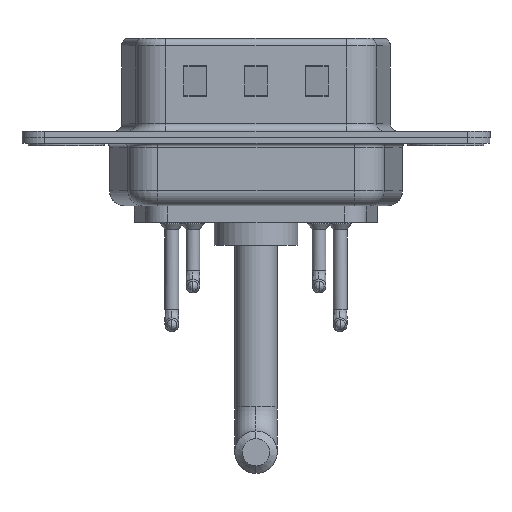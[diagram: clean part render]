
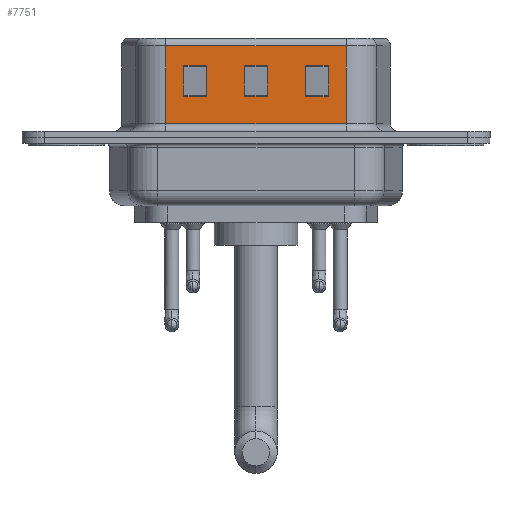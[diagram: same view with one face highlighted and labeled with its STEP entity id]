
A CAD part, front view. The second image highlights one B-rep face of the part: STEP entity #7751.
In plain terms, the highlighted planar face has unit normal (0, -1, 0).
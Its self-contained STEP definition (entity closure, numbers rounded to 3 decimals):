
#421 = FACE_OUTER_BOUND ( 'NONE', #4052, .T. ) ;
#443 = LINE ( 'NONE', #3207, #544 ) ;
#544 = VECTOR ( 'NONE', #8611, 1000. ) ;
#667 = CARTESIAN_POINT ( 'NONE',  ( 7.75, -4.55, 2.705 ) ) ;
#671 = EDGE_CURVE ( 'NONE', #2100, #13648, #8820, .T. ) ;
#687 = DIRECTION ( 'NONE',  ( -1., 0., 0. ) ) ;
#798 = CARTESIAN_POINT ( 'NONE',  ( 11.75, -4.55, 2.705 ) ) ;
#935 = VERTEX_POINT ( 'NONE', #10916 ) ;
#1129 = EDGE_CURVE ( 'NONE', #3249, #13565, #11457, .T. ) ;
#1259 = VECTOR ( 'NONE', #13180, 1000. ) ;
#1276 = CARTESIAN_POINT ( 'NONE',  ( 18.451, -4.55, 6.02 ) ) ;
#1344 = VECTOR ( 'NONE', #3215, 1000. ) ;
#1356 = DIRECTION ( 'NONE',  ( 1., 0., 0. ) ) ;
#1437 = VERTEX_POINT ( 'NONE', #798 ) ;
#1590 = VERTEX_POINT ( 'NONE', #16400 ) ;
#1668 = FACE_BOUND ( 'NONE', #7060, .T. ) ;
#1774 = VERTEX_POINT ( 'NONE', #2992 ) ;
#1890 = EDGE_CURVE ( 'NONE', #15022, #1437, #7708, .T. ) ;
#1891 = EDGE_CURVE ( 'NONE', #13648, #3902, #11852, .T. ) ;
#2100 = VERTEX_POINT ( 'NONE', #8487 ) ;
#2516 = CARTESIAN_POINT ( 'NONE',  ( 14.451, -4.55, 4.705 ) ) ;
#2557 = EDGE_CURVE ( 'NONE', #2567, #9146, #14046, .T. ) ;
#2567 = VERTEX_POINT ( 'NONE', #9972 ) ;
#2642 = ORIENTED_EDGE ( 'NONE', *, *, #10683, .T. ) ;
#2862 = ORIENTED_EDGE ( 'NONE', *, *, #17486, .T. ) ;
#2992 = CARTESIAN_POINT ( 'NONE',  ( 15.75, -4.55, 2.705 ) ) ;
#3095 = CARTESIAN_POINT ( 'NONE',  ( 18.451, -4.55, 6.52 ) ) ;
#3207 = CARTESIAN_POINT ( 'NONE',  ( 18.451, -4.55, 0.9 ) ) ;
#3215 = DIRECTION ( 'NONE',  ( 0., 0., 1. ) ) ;
#3233 = DIRECTION ( 'NONE',  ( 1., 0., 0. ) ) ;
#3249 = VERTEX_POINT ( 'NONE', #9520 ) ;
#3403 = DIRECTION ( 'NONE',  ( 1., 0., 0. ) ) ;
#3591 = VECTOR ( 'NONE', #12811, 1000. ) ;
#3627 = CARTESIAN_POINT ( 'NONE',  ( 18.451, -4.55, 0.9 ) ) ;
#3777 = CARTESIAN_POINT ( 'NONE',  ( 22.451, -4.55, 2.705 ) ) ;
#3902 = VERTEX_POINT ( 'NONE', #11196 ) ;
#4052 = EDGE_LOOP ( 'NONE', ( #14778, #10621, #5900, #13824 ) ) ;
#4196 = VERTEX_POINT ( 'NONE', #8003 ) ;
#4201 = DIRECTION ( 'NONE',  ( 0., 0., -1. ) ) ;
#4216 = ORIENTED_EDGE ( 'NONE', *, *, #14753, .T. ) ;
#4244 = VECTOR ( 'NONE', #3233, 1000. ) ;
#4467 = VECTOR ( 'NONE', #11379, 1000. ) ;
#5243 = DIRECTION ( 'NONE',  ( 0., 0., -1. ) ) ;
#5418 = CARTESIAN_POINT ( 'NONE',  ( 6.549, -4.55, 6.02 ) ) ;
#5514 = LINE ( 'NONE', #2516, #11904 ) ;
#5900 = ORIENTED_EDGE ( 'NONE', *, *, #15663, .T. ) ;
#6039 = ORIENTED_EDGE ( 'NONE', *, *, #11888, .T. ) ;
#6347 = CARTESIAN_POINT ( 'NONE',  ( 11.75, -4.55, 6.52 ) ) ;
#6568 = CARTESIAN_POINT ( 'NONE',  ( 9.25, -4.55, 4.705 ) ) ;
#6750 = CARTESIAN_POINT ( 'NONE',  ( 6.549, -4.55, 6.52 ) ) ;
#6927 = VECTOR ( 'NONE', #687, 1000. ) ;
#7060 = EDGE_LOOP ( 'NONE', ( #4216, #15397, #7158, #9634 ) ) ;
#7158 = ORIENTED_EDGE ( 'NONE', *, *, #12634, .T. ) ;
#7344 = VECTOR ( 'NONE', #10807, 1000. ) ;
#7421 = CARTESIAN_POINT ( 'NONE',  ( 17.25, -4.55, 4.705 ) ) ;
#7506 = ORIENTED_EDGE ( 'NONE', *, *, #9407, .T. ) ;
#7522 = CARTESIAN_POINT ( 'NONE',  ( 13.25, -4.55, 2.705 ) ) ;
#7557 = LINE ( 'NONE', #8884, #10496 ) ;
#7708 = LINE ( 'NONE', #9021, #6927 ) ;
#7721 = EDGE_LOOP ( 'NONE', ( #12800, #2642, #14802, #7990 ) ) ;
#7751 = ADVANCED_FACE ( 'NONE', ( #1668, #12505, #11163, #421 ), #15250, .F. ) ;
#7990 = ORIENTED_EDGE ( 'NONE', *, *, #671, .T. ) ;
#8003 = CARTESIAN_POINT ( 'NONE',  ( 6.549, -4.55, 0.9 ) ) ;
#8182 = VECTOR ( 'NONE', #9176, 1000. ) ;
#8240 = VECTOR ( 'NONE', #5243, 1000. ) ;
#8441 = EDGE_CURVE ( 'NONE', #2567, #12931, #10846, .T. ) ;
#8487 = CARTESIAN_POINT ( 'NONE',  ( 15.75, -4.55, 4.705 ) ) ;
#8512 = DIRECTION ( 'NONE',  ( 0., 1., 0. ) ) ;
#8611 = DIRECTION ( 'NONE',  ( 1., 0., 0. ) ) ;
#8810 = LINE ( 'NONE', #13137, #3591 ) ;
#8820 = LINE ( 'NONE', #9785, #4244 ) ;
#8853 = CARTESIAN_POINT ( 'NONE',  ( 17.25, -4.55, 6.52 ) ) ;
#8868 = ORIENTED_EDGE ( 'NONE', *, *, #1890, .T. ) ;
#8884 = CARTESIAN_POINT ( 'NONE',  ( 18.451, -4.55, 4.705 ) ) ;
#9021 = CARTESIAN_POINT ( 'NONE',  ( 18.451, -4.55, 2.705 ) ) ;
#9146 = VERTEX_POINT ( 'NONE', #3627 ) ;
#9176 = DIRECTION ( 'NONE',  ( -1., 0., 0. ) ) ;
#9396 = LINE ( 'NONE', #13468, #7344 ) ;
#9407 = EDGE_CURVE ( 'NONE', #935, #15022, #16697, .T. ) ;
#9434 = EDGE_CURVE ( 'NONE', #1774, #2100, #12707, .T. ) ;
#9520 = CARTESIAN_POINT ( 'NONE',  ( 9.25, -4.55, 2.705 ) ) ;
#9634 = ORIENTED_EDGE ( 'NONE', *, *, #17117, .T. ) ;
#9785 = CARTESIAN_POINT ( 'NONE',  ( 22.451, -4.55, 4.705 ) ) ;
#9972 = CARTESIAN_POINT ( 'NONE',  ( 18.451, -4.55, 6.02 ) ) ;
#10038 = DIRECTION ( 'NONE',  ( -1., 0., 0. ) ) ;
#10496 = VECTOR ( 'NONE', #3403, 1000. ) ;
#10621 = ORIENTED_EDGE ( 'NONE', *, *, #8441, .T. ) ;
#10683 = EDGE_CURVE ( 'NONE', #3902, #1774, #15940, .T. ) ;
#10807 = DIRECTION ( 'NONE',  ( 0., 0., -1. ) ) ;
#10846 = LINE ( 'NONE', #1276, #16951 ) ;
#10880 = VECTOR ( 'NONE', #10038, 1000. ) ;
#10916 = CARTESIAN_POINT ( 'NONE',  ( 13.25, -4.55, 4.705 ) ) ;
#10940 = EDGE_LOOP ( 'NONE', ( #2862, #7506, #8868, #6039 ) ) ;
#11163 = FACE_BOUND ( 'NONE', #10940, .T. ) ;
#11196 = CARTESIAN_POINT ( 'NONE',  ( 17.25, -4.55, 2.705 ) ) ;
#11258 = AXIS2_PLACEMENT_3D ( 'NONE', #3095, #8512, #13915 ) ;
#11379 = DIRECTION ( 'NONE',  ( 0., 0., -1. ) ) ;
#11457 = LINE ( 'NONE', #16524, #10880 ) ;
#11765 = VERTEX_POINT ( 'NONE', #16564 ) ;
#11852 = LINE ( 'NONE', #8853, #1259 ) ;
#11888 = EDGE_CURVE ( 'NONE', #1437, #1590, #12920, .T. ) ;
#11904 = VECTOR ( 'NONE', #1356, 1000. ) ;
#12505 = FACE_BOUND ( 'NONE', #7721, .T. ) ;
#12616 = CARTESIAN_POINT ( 'NONE',  ( 13.25, -4.55, 6.52 ) ) ;
#12634 = EDGE_CURVE ( 'NONE', #13565, #11765, #8810, .T. ) ;
#12707 = LINE ( 'NONE', #17507, #1344 ) ;
#12800 = ORIENTED_EDGE ( 'NONE', *, *, #1891, .T. ) ;
#12811 = DIRECTION ( 'NONE',  ( 0., 0., 1. ) ) ;
#12920 = LINE ( 'NONE', #6347, #13882 ) ;
#12931 = VERTEX_POINT ( 'NONE', #5418 ) ;
#13137 = CARTESIAN_POINT ( 'NONE',  ( 7.75, -4.55, 6.52 ) ) ;
#13180 = DIRECTION ( 'NONE',  ( 0., 0., -1. ) ) ;
#13468 = CARTESIAN_POINT ( 'NONE',  ( 9.25, -4.55, 6.52 ) ) ;
#13565 = VERTEX_POINT ( 'NONE', #667 ) ;
#13648 = VERTEX_POINT ( 'NONE', #7421 ) ;
#13824 = ORIENTED_EDGE ( 'NONE', *, *, #14482, .T. ) ;
#13882 = VECTOR ( 'NONE', #16917, 1000. ) ;
#13915 = DIRECTION ( 'NONE',  ( -1., 0., 0. ) ) ;
#14029 = VECTOR ( 'NONE', #4201, 1000. ) ;
#14046 = LINE ( 'NONE', #16357, #14029 ) ;
#14482 = EDGE_CURVE ( 'NONE', #4196, #9146, #443, .T. ) ;
#14676 = VERTEX_POINT ( 'NONE', #6568 ) ;
#14753 = EDGE_CURVE ( 'NONE', #14676, #3249, #9396, .T. ) ;
#14778 = ORIENTED_EDGE ( 'NONE', *, *, #2557, .F. ) ;
#14802 = ORIENTED_EDGE ( 'NONE', *, *, #9434, .T. ) ;
#15022 = VERTEX_POINT ( 'NONE', #7522 ) ;
#15250 = PLANE ( 'NONE',  #11258 ) ;
#15281 = DIRECTION ( 'NONE',  ( -1., 0., 0. ) ) ;
#15397 = ORIENTED_EDGE ( 'NONE', *, *, #1129, .T. ) ;
#15663 = EDGE_CURVE ( 'NONE', #12931, #4196, #17476, .T. ) ;
#15940 = LINE ( 'NONE', #3777, #8182 ) ;
#16357 = CARTESIAN_POINT ( 'NONE',  ( 18.451, -4.55, 6.52 ) ) ;
#16400 = CARTESIAN_POINT ( 'NONE',  ( 11.75, -4.55, 4.705 ) ) ;
#16524 = CARTESIAN_POINT ( 'NONE',  ( 14.451, -4.55, 2.705 ) ) ;
#16564 = CARTESIAN_POINT ( 'NONE',  ( 7.75, -4.55, 4.705 ) ) ;
#16697 = LINE ( 'NONE', #12616, #4467 ) ;
#16917 = DIRECTION ( 'NONE',  ( 0., 0., 1. ) ) ;
#16951 = VECTOR ( 'NONE', #15281, 1000. ) ;
#17117 = EDGE_CURVE ( 'NONE', #11765, #14676, #5514, .T. ) ;
#17476 = LINE ( 'NONE', #6750, #8240 ) ;
#17486 = EDGE_CURVE ( 'NONE', #1590, #935, #7557, .T. ) ;
#17507 = CARTESIAN_POINT ( 'NONE',  ( 15.75, -4.55, 6.52 ) ) ;
